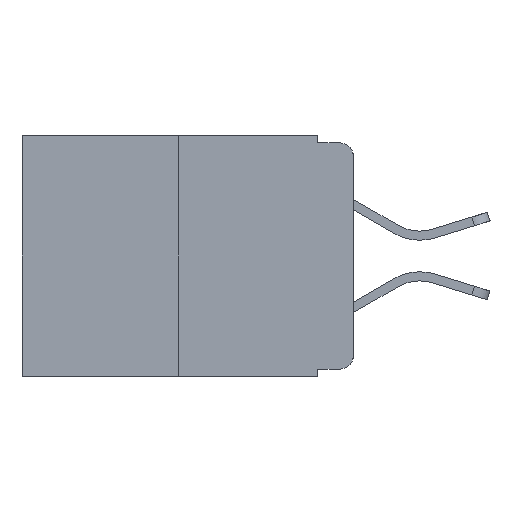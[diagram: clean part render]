
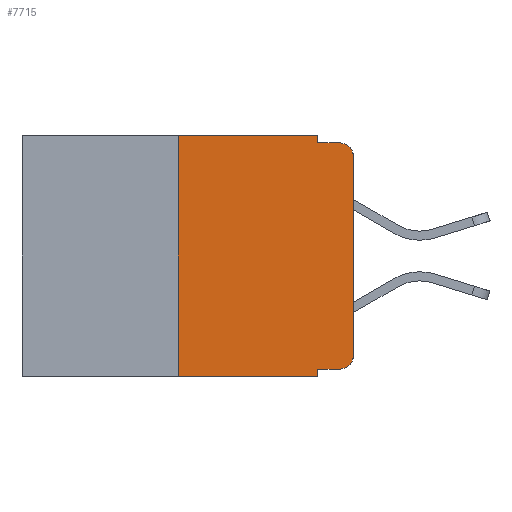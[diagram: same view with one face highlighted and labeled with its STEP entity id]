
A CAD part, left-side view. The second image highlights one B-rep face of the part: STEP entity #7715.
In plain terms, the highlighted planar face has unit normal (-1, 0, 0).
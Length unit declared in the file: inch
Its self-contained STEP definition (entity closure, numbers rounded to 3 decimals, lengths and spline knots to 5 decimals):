
#141 = ORIENTED_EDGE ( 'NONE', *, *, #3900, .F. ) ;
#222 = DIRECTION ( 'NONE',  ( 0., 0., -1. ) ) ;
#299 = ORIENTED_EDGE ( 'NONE', *, *, #12257, .F. ) ;
#538 = EDGE_CURVE ( 'NONE', #10520, #5363, #1251, .T. ) ;
#552 = CARTESIAN_POINT ( 'NONE',  ( 0., 0.473, 0. ) ) ;
#559 = CARTESIAN_POINT ( 'NONE',  ( 0., 0.02, -0.01 ) ) ;
#600 = CARTESIAN_POINT ( 'NONE',  ( 0., 0.051, -0.01 ) ) ;
#762 = VECTOR ( 'NONE', #6959, 39.37008 ) ;
#892 = CARTESIAN_POINT ( 'NONE',  ( 0., 0., -0.313 ) ) ;
#946 = CARTESIAN_POINT ( 'NONE',  ( 0., 0.25, -0.343 ) ) ;
#1171 = LINE ( 'NONE', #3587, #3252 ) ;
#1234 = DIRECTION ( 'NONE',  ( 0., -1., 0. ) ) ;
#1235 = EDGE_CURVE ( 'NONE', #2640, #9174, #3774, .T. ) ;
#1251 = LINE ( 'NONE', #10425, #3935 ) ;
#1274 = EDGE_CURVE ( 'NONE', #3406, #2640, #3468, .T. ) ;
#1544 = ORIENTED_EDGE ( 'NONE', *, *, #538, .T. ) ;
#1562 = DIRECTION ( 'NONE',  ( 0., 0., -1. ) ) ;
#1615 = CARTESIAN_POINT ( 'NONE',  ( 0., 0.25, 0. ) ) ;
#2263 = FACE_OUTER_BOUND ( 'NONE', #8822, .T. ) ;
#2596 = LINE ( 'NONE', #7663, #5194 ) ;
#2640 = VERTEX_POINT ( 'NONE', #11206 ) ;
#2936 = VECTOR ( 'NONE', #4582, 39.37008 ) ;
#3252 = VECTOR ( 'NONE', #3628, 39.37008 ) ;
#3406 = VERTEX_POINT ( 'NONE', #6041 ) ;
#3468 = LINE ( 'NONE', #8556, #762 ) ;
#3587 = CARTESIAN_POINT ( 'NONE',  ( 0., 0.051, 0. ) ) ;
#3628 = DIRECTION ( 'NONE',  ( 0., 0., -1. ) ) ;
#3670 = EDGE_CURVE ( 'NONE', #9174, #7560, #7589, .T. ) ;
#3774 = CIRCLE ( 'NONE', #8665, 0.02 ) ;
#3900 = EDGE_CURVE ( 'NONE', #10520, #5970, #11070, .T. ) ;
#3935 = VECTOR ( 'NONE', #8820, 39.37008 ) ;
#4358 = ORIENTED_EDGE ( 'NONE', *, *, #1274, .T. ) ;
#4537 = PLANE ( 'NONE',  #9959 ) ;
#4582 = DIRECTION ( 'NONE',  ( 0., 0., 1. ) ) ;
#4814 = CIRCLE ( 'NONE', #10539, 0.02 ) ;
#5072 = VECTOR ( 'NONE', #10320, 39.37008 ) ;
#5146 = CARTESIAN_POINT ( 'NONE',  ( 0., 0.051, 0. ) ) ;
#5194 = VECTOR ( 'NONE', #6689, 39.37008 ) ;
#5255 = ORIENTED_EDGE ( 'NONE', *, *, #10536, .F. ) ;
#5321 = CARTESIAN_POINT ( 'NONE',  ( 0., 0.051, -0.343 ) ) ;
#5363 = VERTEX_POINT ( 'NONE', #5321 ) ;
#5507 = DIRECTION ( 'NONE',  ( -1., 0., 0. ) ) ;
#5858 = VERTEX_POINT ( 'NONE', #559 ) ;
#5859 = LINE ( 'NONE', #10583, #8081 ) ;
#5970 = VERTEX_POINT ( 'NONE', #8507 ) ;
#6041 = CARTESIAN_POINT ( 'NONE',  ( 0., 0.051, -0.333 ) ) ;
#6127 = DIRECTION ( 'NONE',  ( -1., 0., 0. ) ) ;
#6151 = CARTESIAN_POINT ( 'NONE',  ( 0., 0.473, 0. ) ) ;
#6451 = ORIENTED_EDGE ( 'NONE', *, *, #7244, .F. ) ;
#6667 = CARTESIAN_POINT ( 'NONE',  ( 0., 0., 0. ) ) ;
#6689 = DIRECTION ( 'NONE',  ( 0., -1., 0. ) ) ;
#6860 = VERTEX_POINT ( 'NONE', #5146 ) ;
#6959 = DIRECTION ( 'NONE',  ( 0., -1., 0. ) ) ;
#7244 = EDGE_CURVE ( 'NONE', #11637, #5858, #2596, .T. ) ;
#7401 = DIRECTION ( 'NONE',  ( 1., 0., 0. ) ) ;
#7560 = VERTEX_POINT ( 'NONE', #11777 ) ;
#7589 = LINE ( 'NONE', #6667, #5072 ) ;
#7663 = CARTESIAN_POINT ( 'NONE',  ( 0., 0.051, -0.01 ) ) ;
#7715 = ADVANCED_FACE ( 'NONE', ( #2263 ), #4537, .F. ) ;
#7786 = DIRECTION ( 'NONE',  ( 0., 0., -1. ) ) ;
#8081 = VECTOR ( 'NONE', #7786, 39.37008 ) ;
#8474 = VECTOR ( 'NONE', #1234, 39.37008 ) ;
#8507 = CARTESIAN_POINT ( 'NONE',  ( 0., 0.25, 0. ) ) ;
#8556 = CARTESIAN_POINT ( 'NONE',  ( 0., 0.051, -0.333 ) ) ;
#8665 = AXIS2_PLACEMENT_3D ( 'NONE', #11709, #6127, #222 ) ;
#8820 = DIRECTION ( 'NONE',  ( 0., -1., 0. ) ) ;
#8822 = EDGE_LOOP ( 'NONE', ( #10120, #9238, #6451, #299, #11844, #141, #1544, #5255, #4358, #11687 ) ) ;
#9174 = VERTEX_POINT ( 'NONE', #892 ) ;
#9238 = ORIENTED_EDGE ( 'NONE', *, *, #10855, .T. ) ;
#9959 = AXIS2_PLACEMENT_3D ( 'NONE', #552, #7401, #1562 ) ;
#10120 = ORIENTED_EDGE ( 'NONE', *, *, #3670, .T. ) ;
#10320 = DIRECTION ( 'NONE',  ( 0., 0., 1. ) ) ;
#10425 = CARTESIAN_POINT ( 'NONE',  ( 0., 0.473, -0.343 ) ) ;
#10520 = VERTEX_POINT ( 'NONE', #946 ) ;
#10536 = EDGE_CURVE ( 'NONE', #3406, #5363, #5859, .T. ) ;
#10539 = AXIS2_PLACEMENT_3D ( 'NONE', #11106, #5507, #12016 ) ;
#10583 = CARTESIAN_POINT ( 'NONE',  ( 0., 0.051, 0. ) ) ;
#10855 = EDGE_CURVE ( 'NONE', #7560, #5858, #4814, .T. ) ;
#10941 = LINE ( 'NONE', #6151, #8474 ) ;
#11070 = LINE ( 'NONE', #1615, #2936 ) ;
#11106 = CARTESIAN_POINT ( 'NONE',  ( 0., 0.02, -0.03 ) ) ;
#11206 = CARTESIAN_POINT ( 'NONE',  ( 0., 0.02, -0.333 ) ) ;
#11637 = VERTEX_POINT ( 'NONE', #600 ) ;
#11687 = ORIENTED_EDGE ( 'NONE', *, *, #1235, .T. ) ;
#11709 = CARTESIAN_POINT ( 'NONE',  ( 0., 0.02, -0.313 ) ) ;
#11777 = CARTESIAN_POINT ( 'NONE',  ( 0., 0., -0.03 ) ) ;
#11844 = ORIENTED_EDGE ( 'NONE', *, *, #12007, .F. ) ;
#12007 = EDGE_CURVE ( 'NONE', #5970, #6860, #10941, .T. ) ;
#12016 = DIRECTION ( 'NONE',  ( 0., 0., -1. ) ) ;
#12257 = EDGE_CURVE ( 'NONE', #6860, #11637, #1171, .T. ) ;
